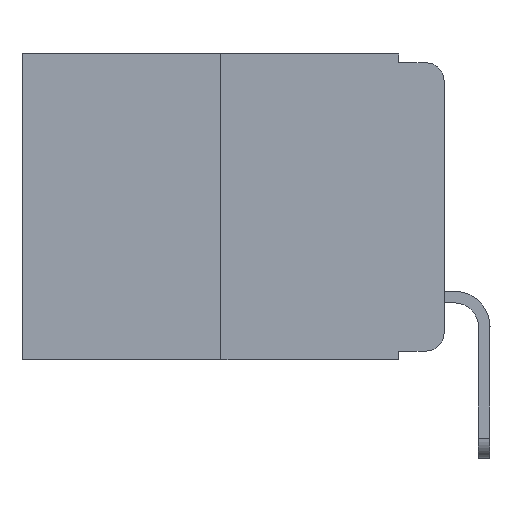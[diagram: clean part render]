
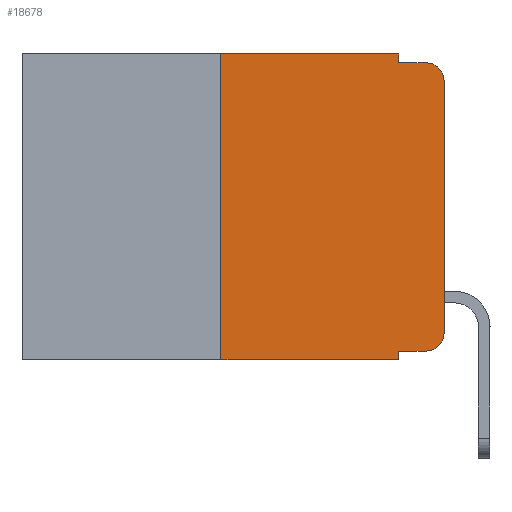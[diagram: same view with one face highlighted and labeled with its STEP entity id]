
A CAD part, left-side view. The second image highlights one B-rep face of the part: STEP entity #18678.
In plain terms, the highlighted planar face has unit normal (-1, 0, 0).
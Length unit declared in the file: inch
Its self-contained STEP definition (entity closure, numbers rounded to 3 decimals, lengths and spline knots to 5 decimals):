
#591 = EDGE_CURVE ( 'NONE', #7695, #22064, #7731, .T. ) ;
#870 = CARTESIAN_POINT ( 'NONE',  ( 0., 0.473, 0. ) ) ;
#1167 = LINE ( 'NONE', #3757, #7416 ) ;
#1516 = DIRECTION ( 'NONE',  ( 0., -1., 0. ) ) ;
#1702 = CARTESIAN_POINT ( 'NONE',  ( 0., 0., -0.03 ) ) ;
#2412 = EDGE_CURVE ( 'NONE', #12160, #7695, #1167, .T. ) ;
#3040 = ORIENTED_EDGE ( 'NONE', *, *, #14150, .F. ) ;
#3757 = CARTESIAN_POINT ( 'NONE',  ( 0., 0.051, 0. ) ) ;
#3772 = LINE ( 'NONE', #15667, #8483 ) ;
#3791 = CARTESIAN_POINT ( 'NONE',  ( 0., 0.051, -0.01 ) ) ;
#3929 = CARTESIAN_POINT ( 'NONE',  ( 0., 0.02, -0.01 ) ) ;
#4101 = CARTESIAN_POINT ( 'NONE',  ( 0., 0.473, 0. ) ) ;
#4547 = LINE ( 'NONE', #16859, #4859 ) ;
#4824 = CARTESIAN_POINT ( 'NONE',  ( 0., 0.02, -0.313 ) ) ;
#4859 = VECTOR ( 'NONE', #15210, 39.37008 ) ;
#4987 = VECTOR ( 'NONE', #5923, 39.37008 ) ;
#5059 = AXIS2_PLACEMENT_3D ( 'NONE', #870, #17537, #7148 ) ;
#5107 = DIRECTION ( 'NONE',  ( 0., 0., -1. ) ) ;
#5316 = CARTESIAN_POINT ( 'NONE',  ( 0., 0.051, -0.333 ) ) ;
#5326 = LINE ( 'NONE', #24345, #24542 ) ;
#5450 = DIRECTION ( 'NONE',  ( 0., 0., 1. ) ) ;
#5877 = DIRECTION ( 'NONE',  ( 0., -1., 0. ) ) ;
#5923 = DIRECTION ( 'NONE',  ( 0., 0., 1. ) ) ;
#6055 = VERTEX_POINT ( 'NONE', #5316 ) ;
#6318 = AXIS2_PLACEMENT_3D ( 'NONE', #8866, #17220, #21994 ) ;
#6391 = AXIS2_PLACEMENT_3D ( 'NONE', #4824, #23825, #5107 ) ;
#6761 = ORIENTED_EDGE ( 'NONE', *, *, #9222, .T. ) ;
#7030 = ORIENTED_EDGE ( 'NONE', *, *, #14652, .T. ) ;
#7148 = DIRECTION ( 'NONE',  ( 0., 0., -1. ) ) ;
#7416 = VECTOR ( 'NONE', #9483, 39.37008 ) ;
#7483 = LINE ( 'NONE', #21727, #21975 ) ;
#7592 = ORIENTED_EDGE ( 'NONE', *, *, #13482, .T. ) ;
#7695 = VERTEX_POINT ( 'NONE', #24917 ) ;
#7731 = LINE ( 'NONE', #3791, #13542 ) ;
#8483 = VECTOR ( 'NONE', #26323, 39.37008 ) ;
#8866 = CARTESIAN_POINT ( 'NONE',  ( 0., 0.02, -0.03 ) ) ;
#9222 = EDGE_CURVE ( 'NONE', #9263, #13118, #5326, .T. ) ;
#9263 = VERTEX_POINT ( 'NONE', #17775 ) ;
#9399 = EDGE_CURVE ( 'NONE', #18161, #12160, #22574, .T. ) ;
#9483 = DIRECTION ( 'NONE',  ( 0., 0., -1. ) ) ;
#9562 = VERTEX_POINT ( 'NONE', #19252 ) ;
#9916 = CARTESIAN_POINT ( 'NONE',  ( 0., 0.051, 0. ) ) ;
#10185 = CIRCLE ( 'NONE', #6318, 0.02 ) ;
#10294 = VERTEX_POINT ( 'NONE', #20855 ) ;
#11259 = FACE_OUTER_BOUND ( 'NONE', #16421, .T. ) ;
#11871 = VECTOR ( 'NONE', #5877, 39.37008 ) ;
#12160 = VERTEX_POINT ( 'NONE', #9916 ) ;
#13118 = VERTEX_POINT ( 'NONE', #20112 ) ;
#13482 = EDGE_CURVE ( 'NONE', #9562, #24523, #7483, .T. ) ;
#13542 = VECTOR ( 'NONE', #17985, 39.37008 ) ;
#14150 = EDGE_CURVE ( 'NONE', #9263, #18161, #24659, .T. ) ;
#14652 = EDGE_CURVE ( 'NONE', #24523, #22064, #10185, .T. ) ;
#15210 = DIRECTION ( 'NONE',  ( 0., -1., 0. ) ) ;
#15570 = CIRCLE ( 'NONE', #6391, 0.02 ) ;
#15667 = CARTESIAN_POINT ( 'NONE',  ( 0., 0.051, 0. ) ) ;
#15696 = EDGE_CURVE ( 'NONE', #6055, #13118, #3772, .T. ) ;
#16312 = ORIENTED_EDGE ( 'NONE', *, *, #20928, .T. ) ;
#16421 = EDGE_LOOP ( 'NONE', ( #7592, #7030, #21795, #17825, #26443, #3040, #6761, #16474, #26999, #16312 ) ) ;
#16474 = ORIENTED_EDGE ( 'NONE', *, *, #15696, .F. ) ;
#16859 = CARTESIAN_POINT ( 'NONE',  ( 0., 0.051, -0.333 ) ) ;
#17220 = DIRECTION ( 'NONE',  ( -1., 0., 0. ) ) ;
#17343 = CARTESIAN_POINT ( 'NONE',  ( 0., 0.25, 0. ) ) ;
#17537 = DIRECTION ( 'NONE',  ( 1., 0., 0. ) ) ;
#17775 = CARTESIAN_POINT ( 'NONE',  ( 0., 0.25, -0.343 ) ) ;
#17825 = ORIENTED_EDGE ( 'NONE', *, *, #2412, .F. ) ;
#17985 = DIRECTION ( 'NONE',  ( 0., -1., 0. ) ) ;
#18161 = VERTEX_POINT ( 'NONE', #17343 ) ;
#18678 = ADVANCED_FACE ( 'NONE', ( #11259 ), #19611, .F. ) ;
#18764 = CARTESIAN_POINT ( 'NONE',  ( 0., 0.25, 0. ) ) ;
#19252 = CARTESIAN_POINT ( 'NONE',  ( 0., 0., -0.313 ) ) ;
#19611 = PLANE ( 'NONE',  #5059 ) ;
#20112 = CARTESIAN_POINT ( 'NONE',  ( 0., 0.051, -0.343 ) ) ;
#20855 = CARTESIAN_POINT ( 'NONE',  ( 0., 0.02, -0.333 ) ) ;
#20928 = EDGE_CURVE ( 'NONE', #10294, #9562, #15570, .T. ) ;
#21727 = CARTESIAN_POINT ( 'NONE',  ( 0., 0., 0. ) ) ;
#21795 = ORIENTED_EDGE ( 'NONE', *, *, #591, .F. ) ;
#21975 = VECTOR ( 'NONE', #5450, 39.37008 ) ;
#21994 = DIRECTION ( 'NONE',  ( 0., 0., -1. ) ) ;
#22064 = VERTEX_POINT ( 'NONE', #3929 ) ;
#22574 = LINE ( 'NONE', #4101, #11871 ) ;
#23463 = EDGE_CURVE ( 'NONE', #6055, #10294, #4547, .T. ) ;
#23825 = DIRECTION ( 'NONE',  ( -1., 0., 0. ) ) ;
#24345 = CARTESIAN_POINT ( 'NONE',  ( 0., 0.473, -0.343 ) ) ;
#24523 = VERTEX_POINT ( 'NONE', #1702 ) ;
#24542 = VECTOR ( 'NONE', #1516, 39.37008 ) ;
#24659 = LINE ( 'NONE', #18764, #4987 ) ;
#24917 = CARTESIAN_POINT ( 'NONE',  ( 0., 0.051, -0.01 ) ) ;
#26323 = DIRECTION ( 'NONE',  ( 0., 0., -1. ) ) ;
#26443 = ORIENTED_EDGE ( 'NONE', *, *, #9399, .F. ) ;
#26999 = ORIENTED_EDGE ( 'NONE', *, *, #23463, .T. ) ;
